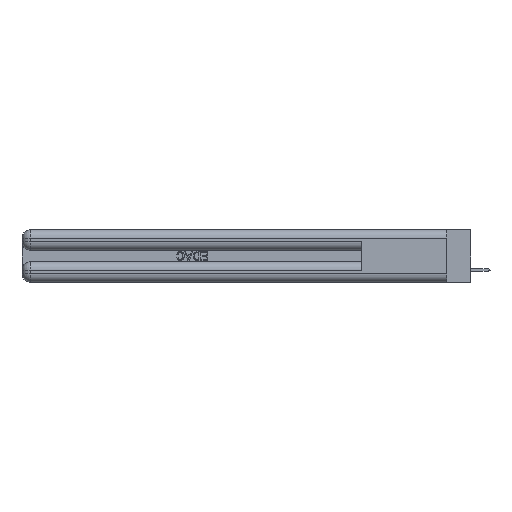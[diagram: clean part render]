
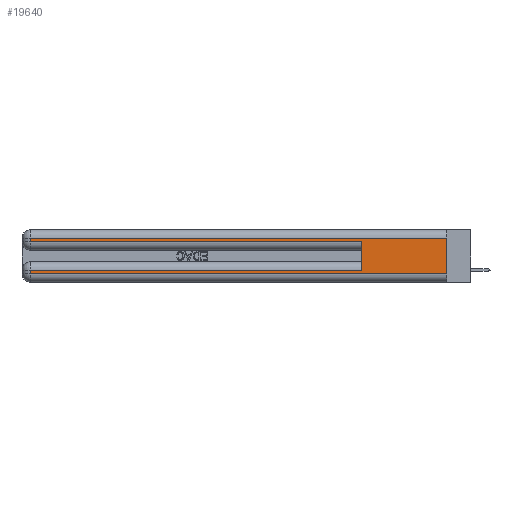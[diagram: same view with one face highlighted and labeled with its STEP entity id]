
A CAD part, left-side view. The second image highlights one B-rep face of the part: STEP entity #19640.
In plain terms, the highlighted planar face has unit normal (-1, 0, 0).
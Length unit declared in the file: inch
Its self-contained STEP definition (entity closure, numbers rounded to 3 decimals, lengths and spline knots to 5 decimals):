
#525 = ORIENTED_EDGE ( 'NONE', *, *, #35186, .T. ) ;
#1039 = VERTEX_POINT ( 'NONE', #37177 ) ;
#1256 = VERTEX_POINT ( 'NONE', #43233 ) ;
#1839 = CARTESIAN_POINT ( 'NONE',  ( 0., 2.94, 0.37 ) ) ;
#1893 = LINE ( 'NONE', #17690, #42013 ) ;
#2570 = DIRECTION ( 'NONE',  ( 0., 1., 0. ) ) ;
#2844 = DIRECTION ( 'NONE',  ( 0., 0., -1. ) ) ;
#3048 = CARTESIAN_POINT ( 'NONE',  ( 0., 0., 0.085 ) ) ;
#3479 = VERTEX_POINT ( 'NONE', #39322 ) ;
#4466 = CARTESIAN_POINT ( 'NONE',  ( 0., 0.6, 0.145 ) ) ;
#4763 = CARTESIAN_POINT ( 'NONE',  ( 0., 0.6, 0.285 ) ) ;
#5023 = VECTOR ( 'NONE', #19310, 39.37008 ) ;
#5455 = LINE ( 'NONE', #25330, #43395 ) ;
#5579 = ORIENTED_EDGE ( 'NONE', *, *, #45619, .F. ) ;
#5584 = CARTESIAN_POINT ( 'NONE',  ( 0., 2.94, 0.37 ) ) ;
#5966 = EDGE_CURVE ( 'NONE', #19258, #3479, #13360, .T. ) ;
#7024 = CARTESIAN_POINT ( 'NONE',  ( 0., 0., 0.285 ) ) ;
#8087 = EDGE_CURVE ( 'NONE', #1039, #36817, #40275, .T. ) ;
#10214 = VECTOR ( 'NONE', #28221, 39.37008 ) ;
#12838 = VERTEX_POINT ( 'NONE', #31256 ) ;
#13360 = LINE ( 'NONE', #5584, #10214 ) ;
#13382 = CARTESIAN_POINT ( 'NONE',  ( 0., 2.94, 0.31 ) ) ;
#13700 = CARTESIAN_POINT ( 'NONE',  ( 0., 0., 0.31 ) ) ;
#15980 = EDGE_CURVE ( 'NONE', #36817, #12838, #24235, .T. ) ;
#16687 = DIRECTION ( 'NONE',  ( 0., 0., -1. ) ) ;
#17644 = ORIENTED_EDGE ( 'NONE', *, *, #19558, .F. ) ;
#17690 = CARTESIAN_POINT ( 'NONE',  ( 0., 0., 0.37 ) ) ;
#19258 = VERTEX_POINT ( 'NONE', #13382 ) ;
#19310 = DIRECTION ( 'NONE',  ( 0., 0., 1. ) ) ;
#19558 = EDGE_CURVE ( 'NONE', #38988, #1256, #1893, .T. ) ;
#19640 = ADVANCED_FACE ( 'NONE', ( #35733 ), #32545, .F. ) ;
#19964 = CARTESIAN_POINT ( 'NONE',  ( 0., 2.94, 0.085 ) ) ;
#20272 = AXIS2_PLACEMENT_3D ( 'NONE', #46434, #42546, #2844 ) ;
#23046 = ORIENTED_EDGE ( 'NONE', *, *, #24352, .T. ) ;
#23213 = LINE ( 'NONE', #4466, #5023 ) ;
#24235 = LINE ( 'NONE', #1839, #30277 ) ;
#24352 = EDGE_CURVE ( 'NONE', #38988, #19258, #26386, .T. ) ;
#24386 = VECTOR ( 'NONE', #2570, 39.37008 ) ;
#25007 = DIRECTION ( 'NONE',  ( 0., 0., -1. ) ) ;
#25330 = CARTESIAN_POINT ( 'NONE',  ( 0., 0., 0.06 ) ) ;
#26386 = LINE ( 'NONE', #41222, #41501 ) ;
#26864 = DIRECTION ( 'NONE',  ( 0., 1., 0. ) ) ;
#28221 = DIRECTION ( 'NONE',  ( 0., 0., -1. ) ) ;
#28480 = ORIENTED_EDGE ( 'NONE', *, *, #15980, .T. ) ;
#28705 = DIRECTION ( 'NONE',  ( 0., -1., 0. ) ) ;
#30277 = VECTOR ( 'NONE', #16687, 39.37008 ) ;
#30974 = EDGE_CURVE ( 'NONE', #12838, #1256, #5455, .T. ) ;
#31256 = CARTESIAN_POINT ( 'NONE',  ( 0., 2.94, 0.06 ) ) ;
#32545 = PLANE ( 'NONE',  #20272 ) ;
#34995 = ORIENTED_EDGE ( 'NONE', *, *, #5966, .T. ) ;
#35055 = ORIENTED_EDGE ( 'NONE', *, *, #8087, .T. ) ;
#35186 = EDGE_CURVE ( 'NONE', #3479, #35856, #36715, .T. ) ;
#35733 = FACE_OUTER_BOUND ( 'NONE', #41135, .T. ) ;
#35856 = VERTEX_POINT ( 'NONE', #4763 ) ;
#36715 = LINE ( 'NONE', #7024, #45725 ) ;
#36817 = VERTEX_POINT ( 'NONE', #19964 ) ;
#37177 = CARTESIAN_POINT ( 'NONE',  ( 0., 0.6, 0.085 ) ) ;
#38988 = VERTEX_POINT ( 'NONE', #13700 ) ;
#39322 = CARTESIAN_POINT ( 'NONE',  ( 0., 2.94, 0.285 ) ) ;
#40275 = LINE ( 'NONE', #3048, #24386 ) ;
#41135 = EDGE_LOOP ( 'NONE', ( #17644, #23046, #34995, #525, #5579, #35055, #28480, #43120 ) ) ;
#41222 = CARTESIAN_POINT ( 'NONE',  ( 0., 0., 0.31 ) ) ;
#41501 = VECTOR ( 'NONE', #26864, 39.37008 ) ;
#42013 = VECTOR ( 'NONE', #25007, 39.37008 ) ;
#42546 = DIRECTION ( 'NONE',  ( 1., 0., 0. ) ) ;
#43120 = ORIENTED_EDGE ( 'NONE', *, *, #30974, .T. ) ;
#43233 = CARTESIAN_POINT ( 'NONE',  ( 0., 0., 0.06 ) ) ;
#43395 = VECTOR ( 'NONE', #46341, 39.37008 ) ;
#45619 = EDGE_CURVE ( 'NONE', #1039, #35856, #23213, .T. ) ;
#45725 = VECTOR ( 'NONE', #28705, 39.37008 ) ;
#46341 = DIRECTION ( 'NONE',  ( 0., -1., 0. ) ) ;
#46434 = CARTESIAN_POINT ( 'NONE',  ( 0., 0., 0.37 ) ) ;
